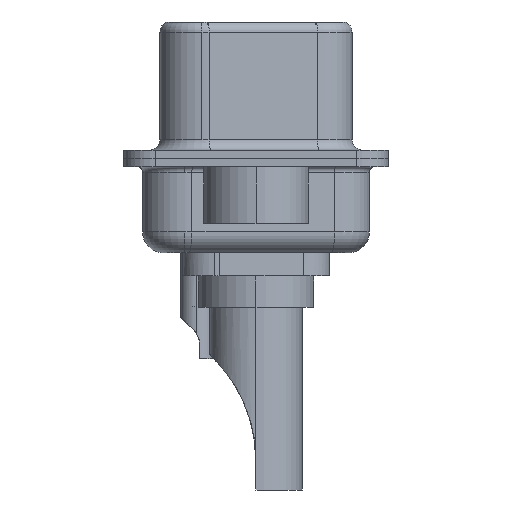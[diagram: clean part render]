
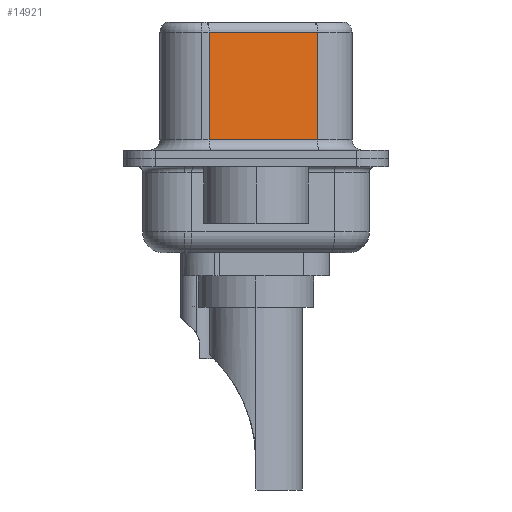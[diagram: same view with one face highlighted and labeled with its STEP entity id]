
A CAD part, left-side view. The second image highlights one B-rep face of the part: STEP entity #14921.
In plain terms, the highlighted planar face has unit normal (-0.985, -0.174, 0).
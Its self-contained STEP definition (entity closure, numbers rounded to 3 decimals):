
#193 = DIRECTION ( 'NONE',  ( -0.174, 0.985, 0. ) ) ;
#712 = VERTEX_POINT ( 'NONE', #19853 ) ;
#757 = VECTOR ( 'NONE', #17320, 1000. ) ;
#2134 = EDGE_LOOP ( 'NONE', ( #9548, #17263, #11505, #20296 ) ) ;
#2714 = VERTEX_POINT ( 'NONE', #19028 ) ;
#3054 = DIRECTION ( 'NONE',  ( 0.985, 0.174, 0. ) ) ;
#3571 = VECTOR ( 'NONE', #193, 1000. ) ;
#3857 = AXIS2_PLACEMENT_3D ( 'NONE', #17333, #3054, #14225 ) ;
#4543 = CARTESIAN_POINT ( 'NONE',  ( 4.58, -2.927, 6.52 ) ) ;
#4619 = CARTESIAN_POINT ( 'NONE',  ( 4.58, -2.927, 0.9 ) ) ;
#4887 = EDGE_CURVE ( 'NONE', #12311, #712, #16815, .T. ) ;
#4967 = LINE ( 'NONE', #4543, #757 ) ;
#5729 = LINE ( 'NONE', #9861, #9444 ) ;
#6431 = DIRECTION ( 'NONE',  ( 0., 0., -1. ) ) ;
#6511 = VECTOR ( 'NONE', #6431, 1000. ) ;
#6669 = FACE_OUTER_BOUND ( 'NONE', #2134, .T. ) ;
#8266 = DIRECTION ( 'NONE',  ( 0.174, -0.985, 0. ) ) ;
#9444 = VECTOR ( 'NONE', #8266, 1000. ) ;
#9548 = ORIENTED_EDGE ( 'NONE', *, *, #13857, .F. ) ;
#9861 = CARTESIAN_POINT ( 'NONE',  ( 4.58, -2.927, 0.9 ) ) ;
#10364 = CARTESIAN_POINT ( 'NONE',  ( 4.58, -2.927, 6.02 ) ) ;
#10517 = CARTESIAN_POINT ( 'NONE',  ( 4.58, -2.927, 6.02 ) ) ;
#10735 = LINE ( 'NONE', #16024, #6511 ) ;
#11505 = ORIENTED_EDGE ( 'NONE', *, *, #18967, .T. ) ;
#12311 = VERTEX_POINT ( 'NONE', #10364 ) ;
#12597 = PLANE ( 'NONE',  #3857 ) ;
#12761 = EDGE_CURVE ( 'NONE', #2714, #14940, #5729, .T. ) ;
#13857 = EDGE_CURVE ( 'NONE', #12311, #14940, #4967, .T. ) ;
#14225 = DIRECTION ( 'NONE',  ( -0.174, 0.985, 0. ) ) ;
#14921 = ADVANCED_FACE ( 'NONE', ( #6669 ), #12597, .F. ) ;
#14940 = VERTEX_POINT ( 'NONE', #4619 ) ;
#16024 = CARTESIAN_POINT ( 'NONE',  ( 3.67, 2.233, 6.52 ) ) ;
#16815 = LINE ( 'NONE', #10517, #3571 ) ;
#17263 = ORIENTED_EDGE ( 'NONE', *, *, #4887, .T. ) ;
#17320 = DIRECTION ( 'NONE',  ( 0., 0., -1. ) ) ;
#17333 = CARTESIAN_POINT ( 'NONE',  ( 4.58, -2.927, 6.52 ) ) ;
#18967 = EDGE_CURVE ( 'NONE', #712, #2714, #10735, .T. ) ;
#19028 = CARTESIAN_POINT ( 'NONE',  ( 3.67, 2.233, 0.9 ) ) ;
#19853 = CARTESIAN_POINT ( 'NONE',  ( 3.67, 2.233, 6.02 ) ) ;
#20296 = ORIENTED_EDGE ( 'NONE', *, *, #12761, .T. ) ;
